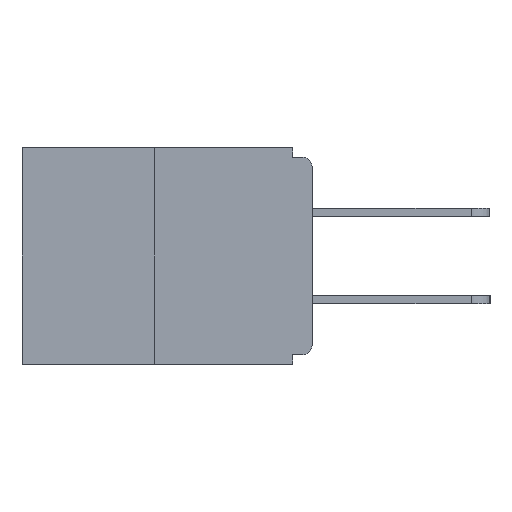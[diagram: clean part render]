
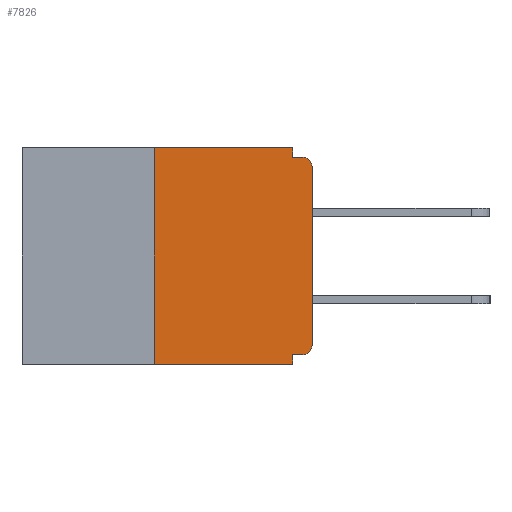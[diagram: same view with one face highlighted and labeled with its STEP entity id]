
A CAD part, left-side view. The second image highlights one B-rep face of the part: STEP entity #7826.
In plain terms, the highlighted planar face has unit normal (-1, 0, 0).
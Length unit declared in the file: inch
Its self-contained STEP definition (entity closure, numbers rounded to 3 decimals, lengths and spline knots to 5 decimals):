
#94 = PLANE ( 'NONE',  #21568 ) ;
#378 = CARTESIAN_POINT ( 'NONE',  ( 0., 0.25, 0. ) ) ;
#753 = VERTEX_POINT ( 'NONE', #5017 ) ;
#756 = EDGE_LOOP ( 'NONE', ( #25027, #26700, #13993, #5357, #26214, #25443, #9694, #13342, #14647, #6379 ) ) ;
#1612 = EDGE_CURVE ( 'NONE', #4237, #24754, #6929, .T. ) ;
#1727 = CARTESIAN_POINT ( 'NONE',  ( 0., 0.031, -0.015 ) ) ;
#1836 = EDGE_CURVE ( 'NONE', #9915, #22064, #10292, .T. ) ;
#1872 = VECTOR ( 'NONE', #11555, 39.37008 ) ;
#1980 = DIRECTION ( 'NONE',  ( 0., 0., -1. ) ) ;
#2283 = CARTESIAN_POINT ( 'NONE',  ( 0., 0.015, -0.328 ) ) ;
#2322 = DIRECTION ( 'NONE',  ( 0., 0., -1. ) ) ;
#2432 = DIRECTION ( 'NONE',  ( 0., 0., -1. ) ) ;
#2612 = DIRECTION ( 'NONE',  ( -1., 0., 0. ) ) ;
#3147 = VECTOR ( 'NONE', #2432, 39.37008 ) ;
#4237 = VERTEX_POINT ( 'NONE', #2283 ) ;
#4332 = CARTESIAN_POINT ( 'NONE',  ( 0., 0., -0.015 ) ) ;
#5017 = CARTESIAN_POINT ( 'NONE',  ( 0., 0.25, 0. ) ) ;
#5357 = ORIENTED_EDGE ( 'NONE', *, *, #13915, .F. ) ;
#6379 = ORIENTED_EDGE ( 'NONE', *, *, #7012, .F. ) ;
#6425 = FACE_OUTER_BOUND ( 'NONE', #756, .T. ) ;
#6929 = CIRCLE ( 'NONE', #16899, 0.015 ) ;
#7012 = EDGE_CURVE ( 'NONE', #11425, #9915, #18646, .T. ) ;
#7826 = ADVANCED_FACE ( 'NONE', ( #6425 ), #94, .F. ) ;
#7888 = CARTESIAN_POINT ( 'NONE',  ( 0., 0.031, 0. ) ) ;
#7917 = CARTESIAN_POINT ( 'NONE',  ( 0., 0.031, -0.328 ) ) ;
#8173 = CARTESIAN_POINT ( 'NONE',  ( 0., 0.46, 0. ) ) ;
#8329 = CARTESIAN_POINT ( 'NONE',  ( 0., 0.46, 0. ) ) ;
#8507 = CARTESIAN_POINT ( 'NONE',  ( 0., 0.031, 0. ) ) ;
#8515 = LINE ( 'NONE', #24869, #23631 ) ;
#8741 = DIRECTION ( 'NONE',  ( 0., 0., 1. ) ) ;
#9694 = ORIENTED_EDGE ( 'NONE', *, *, #24629, .T. ) ;
#9915 = VERTEX_POINT ( 'NONE', #1727 ) ;
#10292 = LINE ( 'NONE', #4332, #14720 ) ;
#10344 = DIRECTION ( 'NONE',  ( 0., -1., 0. ) ) ;
#10573 = CARTESIAN_POINT ( 'NONE',  ( 0., 0.015, -0.03 ) ) ;
#10971 = CARTESIAN_POINT ( 'NONE',  ( 0., 0.031, -0.343 ) ) ;
#11425 = VERTEX_POINT ( 'NONE', #7888 ) ;
#11555 = DIRECTION ( 'NONE',  ( 0., -1., 0. ) ) ;
#11855 = VERTEX_POINT ( 'NONE', #22727 ) ;
#12013 = EDGE_CURVE ( 'NONE', #15099, #22064, #19532, .T. ) ;
#12317 = DIRECTION ( 'NONE',  ( 0., -1., 0. ) ) ;
#13342 = ORIENTED_EDGE ( 'NONE', *, *, #12013, .T. ) ;
#13459 = EDGE_CURVE ( 'NONE', #23105, #753, #19153, .T. ) ;
#13581 = DIRECTION ( 'NONE',  ( 0., 1., 0. ) ) ;
#13839 = LINE ( 'NONE', #25749, #24349 ) ;
#13915 = EDGE_CURVE ( 'NONE', #23140, #11855, #17320, .T. ) ;
#13993 = ORIENTED_EDGE ( 'NONE', *, *, #18048, .T. ) ;
#14647 = ORIENTED_EDGE ( 'NONE', *, *, #1836, .F. ) ;
#14720 = VECTOR ( 'NONE', #12317, 39.37008 ) ;
#14992 = VECTOR ( 'NONE', #10344, 39.37008 ) ;
#15084 = EDGE_CURVE ( 'NONE', #753, #11425, #24270, .T. ) ;
#15099 = VERTEX_POINT ( 'NONE', #24663 ) ;
#15222 = AXIS2_PLACEMENT_3D ( 'NONE', #10573, #23401, #2322 ) ;
#15600 = LINE ( 'NONE', #23844, #1872 ) ;
#15640 = CARTESIAN_POINT ( 'NONE',  ( 0., 0.25, -0.343 ) ) ;
#16193 = DIRECTION ( 'NONE',  ( 1., 0., 0. ) ) ;
#16899 = AXIS2_PLACEMENT_3D ( 'NONE', #23289, #2612, #21534 ) ;
#17164 = CARTESIAN_POINT ( 'NONE',  ( 0., 0., -0.313 ) ) ;
#17320 = LINE ( 'NONE', #10971, #20494 ) ;
#18048 = EDGE_CURVE ( 'NONE', #23105, #11855, #15600, .T. ) ;
#18646 = LINE ( 'NONE', #8507, #3147 ) ;
#19153 = LINE ( 'NONE', #378, #22202 ) ;
#19479 = DIRECTION ( 'NONE',  ( 0., 0., -1. ) ) ;
#19532 = CIRCLE ( 'NONE', #15222, 0.015 ) ;
#20494 = VECTOR ( 'NONE', #19479, 39.37008 ) ;
#20757 = EDGE_CURVE ( 'NONE', #4237, #23140, #13839, .T. ) ;
#21534 = DIRECTION ( 'NONE',  ( 0., 0., -1. ) ) ;
#21568 = AXIS2_PLACEMENT_3D ( 'NONE', #8329, #16193, #1980 ) ;
#22064 = VERTEX_POINT ( 'NONE', #23063 ) ;
#22202 = VECTOR ( 'NONE', #8741, 39.37008 ) ;
#22727 = CARTESIAN_POINT ( 'NONE',  ( 0., 0.031, -0.343 ) ) ;
#23063 = CARTESIAN_POINT ( 'NONE',  ( 0., 0.015, -0.015 ) ) ;
#23105 = VERTEX_POINT ( 'NONE', #15640 ) ;
#23140 = VERTEX_POINT ( 'NONE', #7917 ) ;
#23289 = CARTESIAN_POINT ( 'NONE',  ( 0., 0.015, -0.313 ) ) ;
#23401 = DIRECTION ( 'NONE',  ( -1., 0., 0. ) ) ;
#23631 = VECTOR ( 'NONE', #25008, 39.37008 ) ;
#23844 = CARTESIAN_POINT ( 'NONE',  ( 0., 0.46, -0.343 ) ) ;
#24270 = LINE ( 'NONE', #8173, #14992 ) ;
#24349 = VECTOR ( 'NONE', #13581, 39.37008 ) ;
#24629 = EDGE_CURVE ( 'NONE', #24754, #15099, #8515, .T. ) ;
#24663 = CARTESIAN_POINT ( 'NONE',  ( 0., 0., -0.03 ) ) ;
#24754 = VERTEX_POINT ( 'NONE', #17164 ) ;
#24869 = CARTESIAN_POINT ( 'NONE',  ( 0., 0., 0. ) ) ;
#25008 = DIRECTION ( 'NONE',  ( 0., 0., 1. ) ) ;
#25027 = ORIENTED_EDGE ( 'NONE', *, *, #15084, .F. ) ;
#25443 = ORIENTED_EDGE ( 'NONE', *, *, #1612, .T. ) ;
#25749 = CARTESIAN_POINT ( 'NONE',  ( 0., 0., -0.328 ) ) ;
#26214 = ORIENTED_EDGE ( 'NONE', *, *, #20757, .F. ) ;
#26700 = ORIENTED_EDGE ( 'NONE', *, *, #13459, .F. ) ;
